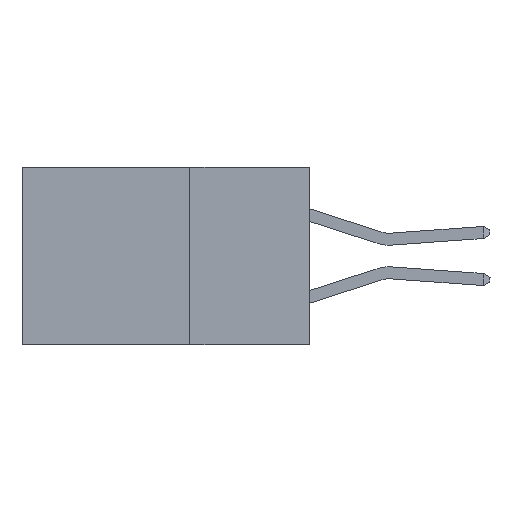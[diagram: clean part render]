
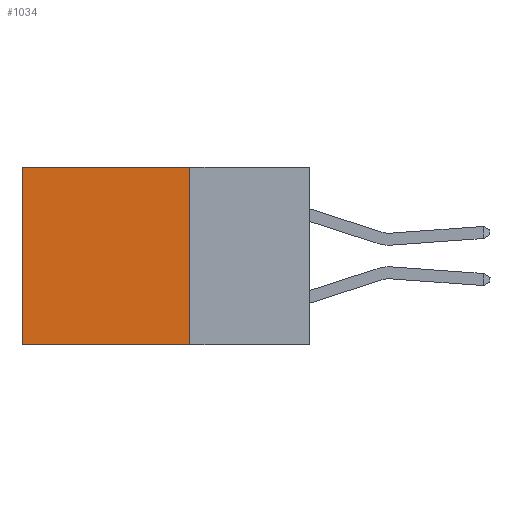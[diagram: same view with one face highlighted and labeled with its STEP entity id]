
A CAD part, left-side view. The second image highlights one B-rep face of the part: STEP entity #1034.
In plain terms, the highlighted planar face has unit normal (-1, 0, 0).
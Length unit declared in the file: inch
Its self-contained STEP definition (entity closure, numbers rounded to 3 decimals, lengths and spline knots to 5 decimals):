
#1034 = ADVANCED_FACE ( 'NONE', ( #1231 ), #2520, .F. ) ;
#1231 = FACE_OUTER_BOUND ( 'NONE', #7907, .T. ) ;
#1325 = ORIENTED_EDGE ( 'NONE', *, *, #5704, .F. ) ;
#1870 = CARTESIAN_POINT ( 'NONE',  ( 0.2615, 0.25, -0.37 ) ) ;
#2211 = DIRECTION ( 'NONE',  ( 1., 0., 0. ) ) ;
#2304 = DIRECTION ( 'NONE',  ( 0., 0., -1. ) ) ;
#2520 = PLANE ( 'NONE',  #12318 ) ;
#3033 = LINE ( 'NONE', #15558, #10369 ) ;
#4000 = CARTESIAN_POINT ( 'NONE',  ( 0.2615, 0.25, 0. ) ) ;
#5261 = ORIENTED_EDGE ( 'NONE', *, *, #9407, .F. ) ;
#5523 = LINE ( 'NONE', #4000, #12320 ) ;
#5704 = EDGE_CURVE ( 'NONE', #16773, #11204, #17741, .T. ) ;
#5852 = CARTESIAN_POINT ( 'NONE',  ( 0.2615, 0.6, -0.37 ) ) ;
#6972 = CARTESIAN_POINT ( 'NONE',  ( 0.2615, 0.6, 0. ) ) ;
#7774 = CARTESIAN_POINT ( 'NONE',  ( 0.2615, 0.25, -0.37 ) ) ;
#7907 = EDGE_LOOP ( 'NONE', ( #11287, #1325, #5261, #17013 ) ) ;
#9048 = CARTESIAN_POINT ( 'NONE',  ( 0.2615, 0.25, -0.37 ) ) ;
#9407 = EDGE_CURVE ( 'NONE', #15130, #16773, #11047, .T. ) ;
#9666 = EDGE_CURVE ( 'NONE', #15869, #11204, #3033, .T. ) ;
#10369 = VECTOR ( 'NONE', #17016, 39.37008 ) ;
#11047 = LINE ( 'NONE', #1870, #18713 ) ;
#11204 = VERTEX_POINT ( 'NONE', #5852 ) ;
#11287 = ORIENTED_EDGE ( 'NONE', *, *, #9666, .T. ) ;
#11330 = CARTESIAN_POINT ( 'NONE',  ( 0.2615, 0.25, -0.37 ) ) ;
#12318 = AXIS2_PLACEMENT_3D ( 'NONE', #7774, #2211, #2304 ) ;
#12320 = VECTOR ( 'NONE', #17085, 39.37008 ) ;
#13545 = DIRECTION ( 'NONE',  ( 0., 0., -1. ) ) ;
#14195 = CARTESIAN_POINT ( 'NONE',  ( 0.2615, 0.25, 0. ) ) ;
#15130 = VERTEX_POINT ( 'NONE', #14195 ) ;
#15558 = CARTESIAN_POINT ( 'NONE',  ( 0.2615, 0.6, -0.37 ) ) ;
#15869 = VERTEX_POINT ( 'NONE', #6972 ) ;
#16773 = VERTEX_POINT ( 'NONE', #9048 ) ;
#17013 = ORIENTED_EDGE ( 'NONE', *, *, #17262, .T. ) ;
#17016 = DIRECTION ( 'NONE',  ( 0., 0., -1. ) ) ;
#17085 = DIRECTION ( 'NONE',  ( 0., 1., 0. ) ) ;
#17262 = EDGE_CURVE ( 'NONE', #15130, #15869, #5523, .T. ) ;
#17288 = VECTOR ( 'NONE', #18579, 39.37008 ) ;
#17741 = LINE ( 'NONE', #11330, #17288 ) ;
#18579 = DIRECTION ( 'NONE',  ( 0., 1., 0. ) ) ;
#18713 = VECTOR ( 'NONE', #13545, 39.37008 ) ;
